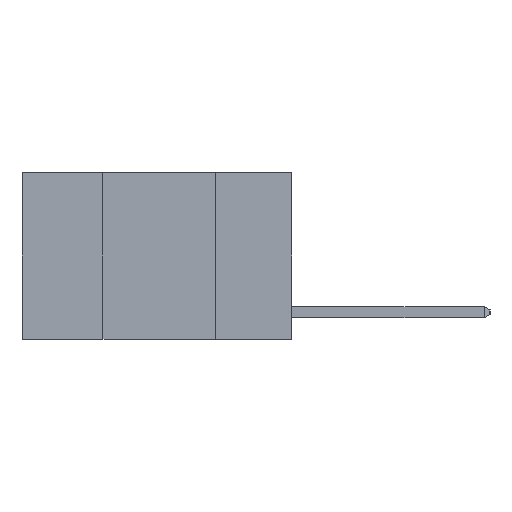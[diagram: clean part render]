
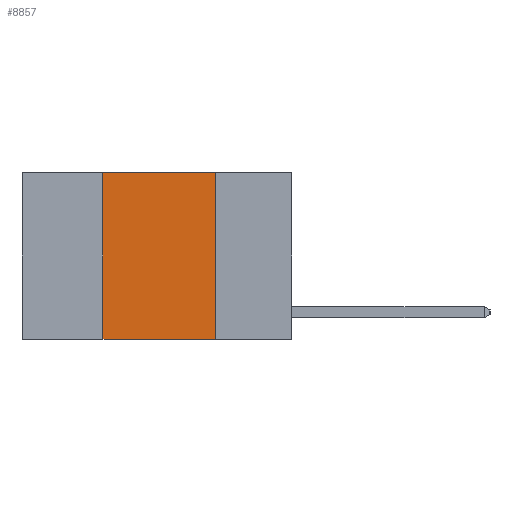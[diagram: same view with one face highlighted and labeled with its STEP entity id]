
A CAD part, left-side view. The second image highlights one B-rep face of the part: STEP entity #8857.
In plain terms, the highlighted planar face has unit normal (-1, 0, 0).
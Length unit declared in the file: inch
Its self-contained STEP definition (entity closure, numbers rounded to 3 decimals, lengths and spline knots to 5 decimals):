
#144 = LINE ( 'NONE', #342, #6226 ) ;
#212 = DIRECTION ( 'NONE',  ( 0., 0., 1. ) ) ;
#342 = CARTESIAN_POINT ( 'NONE',  ( 0., 0.42, 0. ) ) ;
#1369 = VERTEX_POINT ( 'NONE', #1779 ) ;
#1504 = VECTOR ( 'NONE', #2582, 39.37008 ) ;
#1552 = VERTEX_POINT ( 'NONE', #9592 ) ;
#1779 = CARTESIAN_POINT ( 'NONE',  ( 0., 0.42, 0. ) ) ;
#1790 = EDGE_CURVE ( 'NONE', #1552, #1369, #144, .T. ) ;
#1815 = VECTOR ( 'NONE', #2366, 39.37008 ) ;
#1952 = VECTOR ( 'NONE', #5241, 39.37008 ) ;
#2213 = LINE ( 'NONE', #6093, #1952 ) ;
#2366 = DIRECTION ( 'NONE',  ( 0., -1., 0. ) ) ;
#2582 = DIRECTION ( 'NONE',  ( 0., 0., -1. ) ) ;
#3025 = ORIENTED_EDGE ( 'NONE', *, *, #7026, .T. ) ;
#3317 = AXIS2_PLACEMENT_3D ( 'NONE', #9294, #9324, #4470 ) ;
#3687 = PLANE ( 'NONE',  #3317 ) ;
#4470 = DIRECTION ( 'NONE',  ( 0., 0., -1. ) ) ;
#4621 = EDGE_CURVE ( 'NONE', #1369, #9139, #2213, .T. ) ;
#5241 = DIRECTION ( 'NONE',  ( 0., -1., 0. ) ) ;
#5421 = LINE ( 'NONE', #7351, #1504 ) ;
#6064 = ORIENTED_EDGE ( 'NONE', *, *, #1790, .F. ) ;
#6093 = CARTESIAN_POINT ( 'NONE',  ( 0., 0.6, 0. ) ) ;
#6226 = VECTOR ( 'NONE', #212, 39.37008 ) ;
#6739 = FACE_OUTER_BOUND ( 'NONE', #7137, .T. ) ;
#7026 = EDGE_CURVE ( 'NONE', #1552, #9961, #10107, .T. ) ;
#7137 = EDGE_LOOP ( 'NONE', ( #8213, #7768, #6064, #3025 ) ) ;
#7351 = CARTESIAN_POINT ( 'NONE',  ( 0., 0.17, 0. ) ) ;
#7390 = CARTESIAN_POINT ( 'NONE',  ( 0., 0.17, -0.37 ) ) ;
#7768 = ORIENTED_EDGE ( 'NONE', *, *, #4621, .F. ) ;
#8213 = ORIENTED_EDGE ( 'NONE', *, *, #9924, .F. ) ;
#8857 = ADVANCED_FACE ( 'NONE', ( #6739 ), #3687, .F. ) ;
#9139 = VERTEX_POINT ( 'NONE', #9690 ) ;
#9294 = CARTESIAN_POINT ( 'NONE',  ( 0., 0.6, 0. ) ) ;
#9324 = DIRECTION ( 'NONE',  ( 1., 0., 0. ) ) ;
#9592 = CARTESIAN_POINT ( 'NONE',  ( 0., 0.42, -0.37 ) ) ;
#9594 = CARTESIAN_POINT ( 'NONE',  ( 0., 0.6, -0.37 ) ) ;
#9690 = CARTESIAN_POINT ( 'NONE',  ( 0., 0.17, 0. ) ) ;
#9924 = EDGE_CURVE ( 'NONE', #9139, #9961, #5421, .T. ) ;
#9961 = VERTEX_POINT ( 'NONE', #7390 ) ;
#10107 = LINE ( 'NONE', #9594, #1815 ) ;
